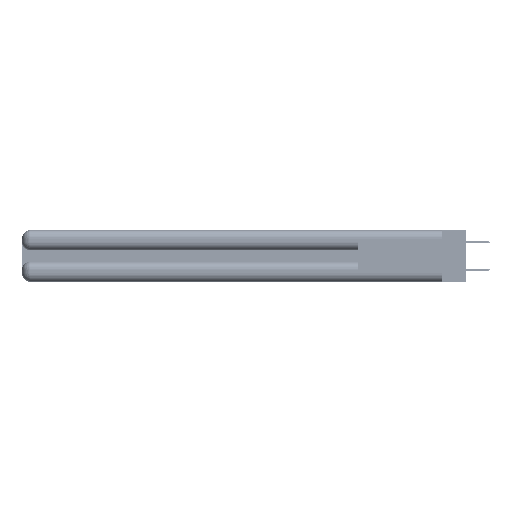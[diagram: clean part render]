
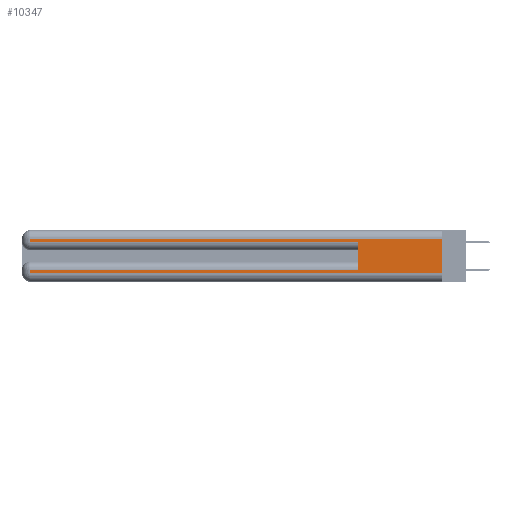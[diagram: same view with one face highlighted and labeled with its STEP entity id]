
A CAD part, left-side view. The second image highlights one B-rep face of the part: STEP entity #10347.
In plain terms, the highlighted planar face has unit normal (-1, 0, 0).
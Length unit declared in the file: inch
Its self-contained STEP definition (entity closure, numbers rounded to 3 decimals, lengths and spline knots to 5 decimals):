
#712 = DIRECTION ( 'NONE',  ( 0., 0., -1. ) ) ;
#1795 = ORIENTED_EDGE ( 'NONE', *, *, #5394, .F. ) ;
#2108 = VECTOR ( 'NONE', #4823, 39.37008 ) ;
#3752 = LINE ( 'NONE', #19852, #14000 ) ;
#4024 = LINE ( 'NONE', #53917, #14291 ) ;
#4497 = CARTESIAN_POINT ( 'NONE',  ( 0., 0., 0.06 ) ) ;
#4823 = DIRECTION ( 'NONE',  ( 0., 0., 1. ) ) ;
#4907 = CARTESIAN_POINT ( 'NONE',  ( 0., 2.94, 0.085 ) ) ;
#5394 = EDGE_CURVE ( 'NONE', #15875, #5425, #36933, .T. ) ;
#5425 = VERTEX_POINT ( 'NONE', #9402 ) ;
#5752 = VECTOR ( 'NONE', #43464, 39.37008 ) ;
#7123 = LINE ( 'NONE', #47824, #5752 ) ;
#7395 = LINE ( 'NONE', #22063, #40914 ) ;
#8880 = DIRECTION ( 'NONE',  ( 0., -1., 0. ) ) ;
#9402 = CARTESIAN_POINT ( 'NONE',  ( 0., 0.6, 0.285 ) ) ;
#9471 = EDGE_CURVE ( 'NONE', #54106, #47365, #28345, .T. ) ;
#10347 = ADVANCED_FACE ( 'NONE', ( #11141 ), #19304, .F. ) ;
#11141 = FACE_OUTER_BOUND ( 'NONE', #44867, .T. ) ;
#11168 = ORIENTED_EDGE ( 'NONE', *, *, #53821, .T. ) ;
#13094 = EDGE_CURVE ( 'NONE', #31432, #47365, #4024, .T. ) ;
#13129 = LINE ( 'NONE', #22248, #55591 ) ;
#14000 = VECTOR ( 'NONE', #37218, 39.37008 ) ;
#14291 = VECTOR ( 'NONE', #45066, 39.37008 ) ;
#15875 = VERTEX_POINT ( 'NONE', #24453 ) ;
#16784 = VERTEX_POINT ( 'NONE', #4907 ) ;
#17387 = LINE ( 'NONE', #48031, #27628 ) ;
#17481 = DIRECTION ( 'NONE',  ( 0., 1., 0. ) ) ;
#19304 = PLANE ( 'NONE',  #20922 ) ;
#19666 = VERTEX_POINT ( 'NONE', #40028 ) ;
#19852 = CARTESIAN_POINT ( 'NONE',  ( 0., 0., 0.285 ) ) ;
#20922 = AXIS2_PLACEMENT_3D ( 'NONE', #45468, #23673, #54331 ) ;
#20940 = ORIENTED_EDGE ( 'NONE', *, *, #33586, .T. ) ;
#21434 = VERTEX_POINT ( 'NONE', #50734 ) ;
#22063 = CARTESIAN_POINT ( 'NONE',  ( 0., 0., 0.085 ) ) ;
#22240 = ORIENTED_EDGE ( 'NONE', *, *, #9471, .T. ) ;
#22248 = CARTESIAN_POINT ( 'NONE',  ( 0., 2.94, 0.37 ) ) ;
#23673 = DIRECTION ( 'NONE',  ( 1., 0., 0. ) ) ;
#24453 = CARTESIAN_POINT ( 'NONE',  ( 0., 0.6, 0.085 ) ) ;
#25628 = ORIENTED_EDGE ( 'NONE', *, *, #38680, .T. ) ;
#25883 = EDGE_CURVE ( 'NONE', #15875, #16784, #7395, .T. ) ;
#26992 = VECTOR ( 'NONE', #8880, 39.37008 ) ;
#27628 = VECTOR ( 'NONE', #17481, 39.37008 ) ;
#28345 = LINE ( 'NONE', #4497, #26992 ) ;
#29721 = CARTESIAN_POINT ( 'NONE',  ( 0., 0., 0.06 ) ) ;
#31432 = VERTEX_POINT ( 'NONE', #56217 ) ;
#33586 = EDGE_CURVE ( 'NONE', #21434, #19666, #7123, .T. ) ;
#36933 = LINE ( 'NONE', #39570, #2108 ) ;
#37218 = DIRECTION ( 'NONE',  ( 0., -1., 0. ) ) ;
#38680 = EDGE_CURVE ( 'NONE', #19666, #5425, #3752, .T. ) ;
#39570 = CARTESIAN_POINT ( 'NONE',  ( 0., 0.6, 0.145 ) ) ;
#40028 = CARTESIAN_POINT ( 'NONE',  ( 0., 2.94, 0.285 ) ) ;
#40914 = VECTOR ( 'NONE', #44061, 39.37008 ) ;
#42235 = ORIENTED_EDGE ( 'NONE', *, *, #13094, .F. ) ;
#43464 = DIRECTION ( 'NONE',  ( 0., 0., -1. ) ) ;
#44061 = DIRECTION ( 'NONE',  ( 0., 1., 0. ) ) ;
#44867 = EDGE_LOOP ( 'NONE', ( #42235, #55594, #20940, #25628, #1795, #55966, #11168, #22240 ) ) ;
#45066 = DIRECTION ( 'NONE',  ( 0., 0., -1. ) ) ;
#45468 = CARTESIAN_POINT ( 'NONE',  ( 0., 0., 0.37 ) ) ;
#46048 = EDGE_CURVE ( 'NONE', #31432, #21434, #17387, .T. ) ;
#46291 = CARTESIAN_POINT ( 'NONE',  ( 0., 2.94, 0.06 ) ) ;
#47365 = VERTEX_POINT ( 'NONE', #29721 ) ;
#47824 = CARTESIAN_POINT ( 'NONE',  ( 0., 2.94, 0.37 ) ) ;
#48031 = CARTESIAN_POINT ( 'NONE',  ( 0., 0., 0.31 ) ) ;
#50734 = CARTESIAN_POINT ( 'NONE',  ( 0., 2.94, 0.31 ) ) ;
#53821 = EDGE_CURVE ( 'NONE', #16784, #54106, #13129, .T. ) ;
#53917 = CARTESIAN_POINT ( 'NONE',  ( 0., 0., 0.37 ) ) ;
#54106 = VERTEX_POINT ( 'NONE', #46291 ) ;
#54331 = DIRECTION ( 'NONE',  ( 0., 0., -1. ) ) ;
#55591 = VECTOR ( 'NONE', #712, 39.37008 ) ;
#55594 = ORIENTED_EDGE ( 'NONE', *, *, #46048, .T. ) ;
#55966 = ORIENTED_EDGE ( 'NONE', *, *, #25883, .T. ) ;
#56217 = CARTESIAN_POINT ( 'NONE',  ( 0., 0., 0.31 ) ) ;
